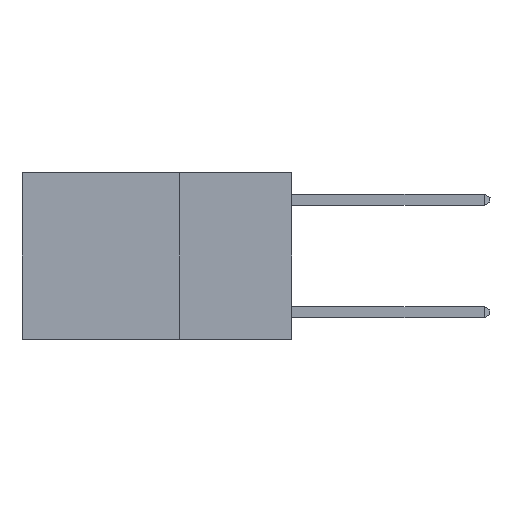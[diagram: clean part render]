
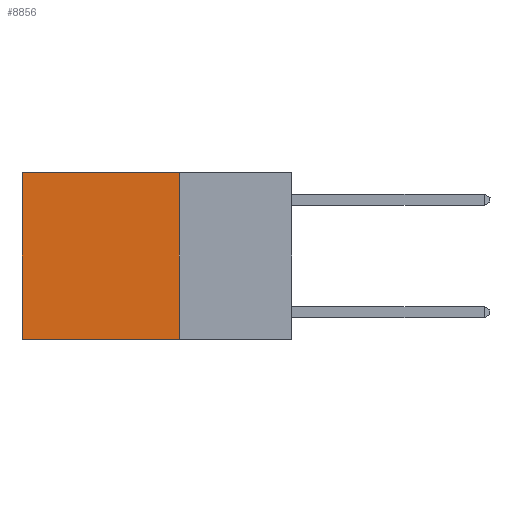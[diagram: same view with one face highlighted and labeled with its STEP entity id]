
A CAD part, left-side view. The second image highlights one B-rep face of the part: STEP entity #8856.
In plain terms, the highlighted planar face has unit normal (-1, 0, 0).
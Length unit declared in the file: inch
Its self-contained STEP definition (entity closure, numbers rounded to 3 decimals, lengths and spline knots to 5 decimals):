
#317 = AXIS2_PLACEMENT_3D ( 'NONE', #9083, #6869, #3939 ) ;
#459 = LINE ( 'NONE', #4019, #8247 ) ;
#817 = EDGE_LOOP ( 'NONE', ( #7690, #2435, #4036, #8072 ) ) ;
#879 = DIRECTION ( 'NONE',  ( 0., 0., -1. ) ) ;
#902 = VECTOR ( 'NONE', #3127, 39.37008 ) ;
#934 = VERTEX_POINT ( 'NONE', #3950 ) ;
#1345 = EDGE_CURVE ( 'NONE', #5003, #9736, #459, .T. ) ;
#1532 = CARTESIAN_POINT ( 'NONE',  ( 0.2625, 0.6, 0. ) ) ;
#1585 = LINE ( 'NONE', #2381, #6043 ) ;
#1772 = VERTEX_POINT ( 'NONE', #2344 ) ;
#2344 = CARTESIAN_POINT ( 'NONE',  ( 0.2625, 0.25, -0.37 ) ) ;
#2381 = CARTESIAN_POINT ( 'NONE',  ( 0.2625, 0.25, 0. ) ) ;
#2435 = ORIENTED_EDGE ( 'NONE', *, *, #5886, .F. ) ;
#2453 = LINE ( 'NONE', #2556, #7811 ) ;
#2533 = CARTESIAN_POINT ( 'NONE',  ( 0.2625, 0.25, 0. ) ) ;
#2556 = CARTESIAN_POINT ( 'NONE',  ( 0.2625, 0.25, -0.37 ) ) ;
#3127 = DIRECTION ( 'NONE',  ( 0., 0., -1. ) ) ;
#3198 = FACE_OUTER_BOUND ( 'NONE', #817, .T. ) ;
#3916 = CARTESIAN_POINT ( 'NONE',  ( 0.2625, 0.6, 0. ) ) ;
#3939 = DIRECTION ( 'NONE',  ( 0., 0., -1. ) ) ;
#3950 = CARTESIAN_POINT ( 'NONE',  ( 0.2625, 0.6, -0.37 ) ) ;
#4019 = CARTESIAN_POINT ( 'NONE',  ( 0.2625, 0.25, 0. ) ) ;
#4036 = ORIENTED_EDGE ( 'NONE', *, *, #4958, .F. ) ;
#4441 = LINE ( 'NONE', #1532, #902 ) ;
#4958 = EDGE_CURVE ( 'NONE', #5003, #1772, #1585, .T. ) ;
#5003 = VERTEX_POINT ( 'NONE', #2533 ) ;
#5642 = DIRECTION ( 'NONE',  ( 0., 1., 0. ) ) ;
#5886 = EDGE_CURVE ( 'NONE', #1772, #934, #2453, .T. ) ;
#6043 = VECTOR ( 'NONE', #879, 39.37008 ) ;
#6591 = EDGE_CURVE ( 'NONE', #9736, #934, #4441, .T. ) ;
#6869 = DIRECTION ( 'NONE',  ( 1., 0., 0. ) ) ;
#7690 = ORIENTED_EDGE ( 'NONE', *, *, #6591, .T. ) ;
#7811 = VECTOR ( 'NONE', #9322, 39.37008 ) ;
#8072 = ORIENTED_EDGE ( 'NONE', *, *, #1345, .T. ) ;
#8247 = VECTOR ( 'NONE', #5642, 39.37008 ) ;
#8380 = PLANE ( 'NONE',  #317 ) ;
#8856 = ADVANCED_FACE ( 'NONE', ( #3198 ), #8380, .F. ) ;
#9083 = CARTESIAN_POINT ( 'NONE',  ( 0.2625, 0.25, 0. ) ) ;
#9322 = DIRECTION ( 'NONE',  ( 0., 1., 0. ) ) ;
#9736 = VERTEX_POINT ( 'NONE', #3916 ) ;
